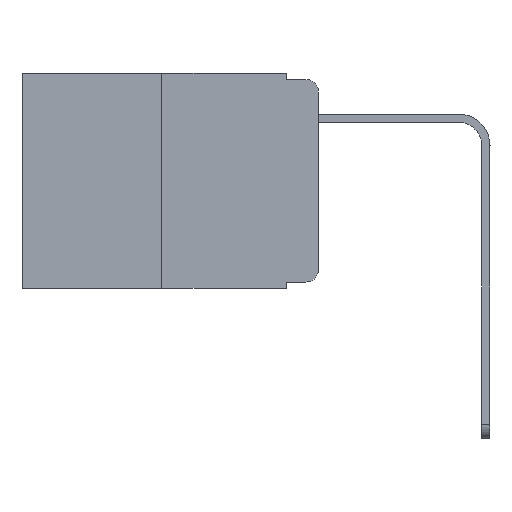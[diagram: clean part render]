
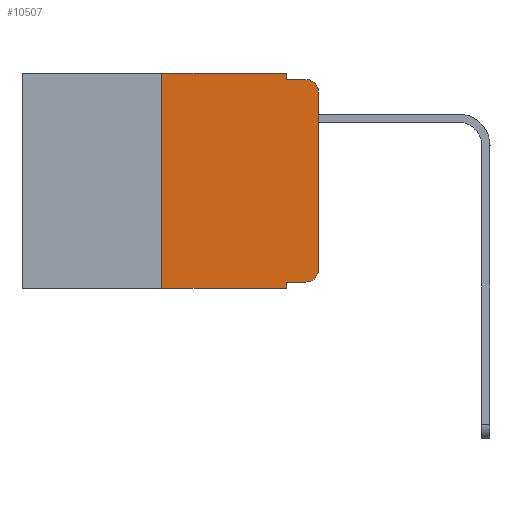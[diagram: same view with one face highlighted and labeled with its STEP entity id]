
A CAD part, left-side view. The second image highlights one B-rep face of the part: STEP entity #10507.
In plain terms, the highlighted planar face has unit normal (-1, 0, 0).
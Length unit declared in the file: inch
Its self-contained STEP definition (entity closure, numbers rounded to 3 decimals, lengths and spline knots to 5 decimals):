
#277 = DIRECTION ( 'NONE',  ( -1., 0., 0. ) ) ;
#668 = CARTESIAN_POINT ( 'NONE',  ( 0., 0.051, -0.343 ) ) ;
#1231 = FACE_OUTER_BOUND ( 'NONE', #21383, .T. ) ;
#1477 = CARTESIAN_POINT ( 'NONE',  ( 0., 0.473, 0. ) ) ;
#1652 = CARTESIAN_POINT ( 'NONE',  ( 0., 0.473, -0.343 ) ) ;
#1668 = CARTESIAN_POINT ( 'NONE',  ( 0., 0., -0.03 ) ) ;
#1737 = AXIS2_PLACEMENT_3D ( 'NONE', #8442, #277, #2116 ) ;
#1813 = VECTOR ( 'NONE', #3001, 39.37008 ) ;
#2035 = ORIENTED_EDGE ( 'NONE', *, *, #19974, .T. ) ;
#2116 = DIRECTION ( 'NONE',  ( 0., 0., -1. ) ) ;
#2376 = AXIS2_PLACEMENT_3D ( 'NONE', #21334, #8959, #5041 ) ;
#3001 = DIRECTION ( 'NONE',  ( 0., 0., 1. ) ) ;
#3298 = AXIS2_PLACEMENT_3D ( 'NONE', #1477, #11626, #16183 ) ;
#3325 = CARTESIAN_POINT ( 'NONE',  ( 0., 0.02, -0.01 ) ) ;
#4117 = VECTOR ( 'NONE', #22911, 39.37008 ) ;
#4463 = EDGE_CURVE ( 'NONE', #16997, #5036, #19457, .T. ) ;
#4691 = LINE ( 'NONE', #16772, #21784 ) ;
#4877 = DIRECTION ( 'NONE',  ( 0., 0., 1. ) ) ;
#5036 = VERTEX_POINT ( 'NONE', #3325 ) ;
#5041 = DIRECTION ( 'NONE',  ( 0., 0., -1. ) ) ;
#5749 = DIRECTION ( 'NONE',  ( 0., -1., 0. ) ) ;
#5855 = CIRCLE ( 'NONE', #1737, 0.02 ) ;
#6306 = VERTEX_POINT ( 'NONE', #7251 ) ;
#7251 = CARTESIAN_POINT ( 'NONE',  ( 0., 0.02, -0.333 ) ) ;
#7620 = VERTEX_POINT ( 'NONE', #668 ) ;
#7691 = CARTESIAN_POINT ( 'NONE',  ( 0., 0.473, 0. ) ) ;
#8442 = CARTESIAN_POINT ( 'NONE',  ( 0., 0.02, -0.03 ) ) ;
#8647 = ORIENTED_EDGE ( 'NONE', *, *, #17013, .T. ) ;
#8959 = DIRECTION ( 'NONE',  ( -1., 0., 0. ) ) ;
#9286 = ORIENTED_EDGE ( 'NONE', *, *, #24408, .F. ) ;
#9289 = DIRECTION ( 'NONE',  ( 0., -1., 0. ) ) ;
#9427 = LINE ( 'NONE', #7691, #15425 ) ;
#10507 = ADVANCED_FACE ( 'NONE', ( #1231 ), #18132, .F. ) ;
#10524 = ORIENTED_EDGE ( 'NONE', *, *, #17795, .T. ) ;
#10836 = CARTESIAN_POINT ( 'NONE',  ( 0., 0.25, 0. ) ) ;
#11399 = LINE ( 'NONE', #1652, #25654 ) ;
#11626 = DIRECTION ( 'NONE',  ( 1., 0., 0. ) ) ;
#12177 = DIRECTION ( 'NONE',  ( 0., -1., 0. ) ) ;
#12232 = VECTOR ( 'NONE', #12177, 39.37008 ) ;
#12257 = EDGE_CURVE ( 'NONE', #17792, #25690, #9427, .T. ) ;
#12479 = VERTEX_POINT ( 'NONE', #24691 ) ;
#12947 = ORIENTED_EDGE ( 'NONE', *, *, #4463, .F. ) ;
#13022 = DIRECTION ( 'NONE',  ( 0., -1., 0. ) ) ;
#14767 = VERTEX_POINT ( 'NONE', #23882 ) ;
#15095 = CARTESIAN_POINT ( 'NONE',  ( 0., 0.051, 0. ) ) ;
#15425 = VECTOR ( 'NONE', #9289, 39.37008 ) ;
#16183 = DIRECTION ( 'NONE',  ( 0., 0., -1. ) ) ;
#16264 = ORIENTED_EDGE ( 'NONE', *, *, #17229, .T. ) ;
#16772 = CARTESIAN_POINT ( 'NONE',  ( 0., 0.051, -0.333 ) ) ;
#16794 = LINE ( 'NONE', #24697, #24418 ) ;
#16807 = CARTESIAN_POINT ( 'NONE',  ( 0., 0.051, 0. ) ) ;
#16887 = LINE ( 'NONE', #10836, #22935 ) ;
#16997 = VERTEX_POINT ( 'NONE', #23819 ) ;
#17013 = EDGE_CURVE ( 'NONE', #14767, #7620, #11399, .T. ) ;
#17020 = LINE ( 'NONE', #25175, #1813 ) ;
#17031 = CARTESIAN_POINT ( 'NONE',  ( 0., 0.25, 0. ) ) ;
#17229 = EDGE_CURVE ( 'NONE', #6306, #12479, #20573, .T. ) ;
#17792 = VERTEX_POINT ( 'NONE', #17031 ) ;
#17795 = EDGE_CURVE ( 'NONE', #23378, #6306, #4691, .T. ) ;
#18132 = PLANE ( 'NONE',  #3298 ) ;
#19457 = LINE ( 'NONE', #24294, #12232 ) ;
#19974 = EDGE_CURVE ( 'NONE', #25421, #5036, #5855, .T. ) ;
#20355 = ORIENTED_EDGE ( 'NONE', *, *, #12257, .F. ) ;
#20573 = CIRCLE ( 'NONE', #2376, 0.02 ) ;
#20693 = DIRECTION ( 'NONE',  ( 0., 0., -1. ) ) ;
#20926 = LINE ( 'NONE', #15095, #4117 ) ;
#21334 = CARTESIAN_POINT ( 'NONE',  ( 0., 0.02, -0.313 ) ) ;
#21383 = EDGE_LOOP ( 'NONE', ( #24051, #2035, #12947, #9286, #20355, #23316, #8647, #24982, #10524, #16264 ) ) ;
#21784 = VECTOR ( 'NONE', #13022, 39.37008 ) ;
#21971 = EDGE_CURVE ( 'NONE', #14767, #17792, #16887, .T. ) ;
#22911 = DIRECTION ( 'NONE',  ( 0., 0., -1. ) ) ;
#22935 = VECTOR ( 'NONE', #4877, 39.37008 ) ;
#23316 = ORIENTED_EDGE ( 'NONE', *, *, #21971, .F. ) ;
#23378 = VERTEX_POINT ( 'NONE', #24195 ) ;
#23819 = CARTESIAN_POINT ( 'NONE',  ( 0., 0.051, -0.01 ) ) ;
#23882 = CARTESIAN_POINT ( 'NONE',  ( 0., 0.25, -0.343 ) ) ;
#24051 = ORIENTED_EDGE ( 'NONE', *, *, #25750, .T. ) ;
#24195 = CARTESIAN_POINT ( 'NONE',  ( 0., 0.051, -0.333 ) ) ;
#24294 = CARTESIAN_POINT ( 'NONE',  ( 0., 0.051, -0.01 ) ) ;
#24408 = EDGE_CURVE ( 'NONE', #25690, #16997, #20926, .T. ) ;
#24418 = VECTOR ( 'NONE', #20693, 39.37008 ) ;
#24564 = EDGE_CURVE ( 'NONE', #23378, #7620, #16794, .T. ) ;
#24691 = CARTESIAN_POINT ( 'NONE',  ( 0., 0., -0.313 ) ) ;
#24697 = CARTESIAN_POINT ( 'NONE',  ( 0., 0.051, 0. ) ) ;
#24982 = ORIENTED_EDGE ( 'NONE', *, *, #24564, .F. ) ;
#25175 = CARTESIAN_POINT ( 'NONE',  ( 0., 0., 0. ) ) ;
#25421 = VERTEX_POINT ( 'NONE', #1668 ) ;
#25654 = VECTOR ( 'NONE', #5749, 39.37008 ) ;
#25690 = VERTEX_POINT ( 'NONE', #16807 ) ;
#25750 = EDGE_CURVE ( 'NONE', #12479, #25421, #17020, .T. ) ;
